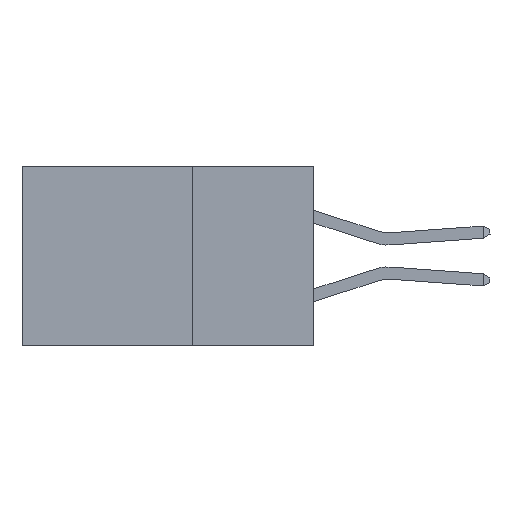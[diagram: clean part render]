
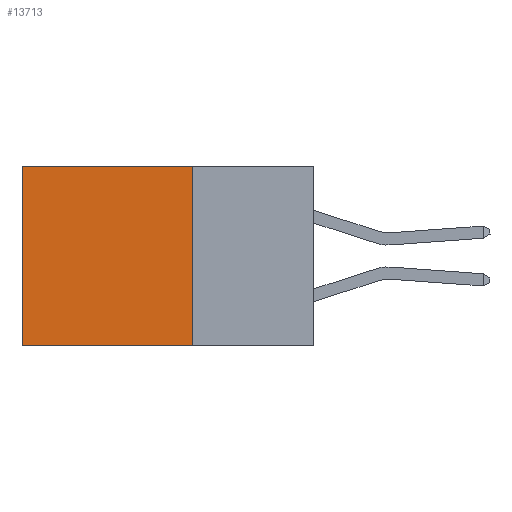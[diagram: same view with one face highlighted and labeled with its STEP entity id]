
A CAD part, left-side view. The second image highlights one B-rep face of the part: STEP entity #13713.
In plain terms, the highlighted planar face has unit normal (-1, 0, 0).
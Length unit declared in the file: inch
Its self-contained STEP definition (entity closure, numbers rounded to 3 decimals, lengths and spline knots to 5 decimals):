
#926 = AXIS2_PLACEMENT_3D ( 'NONE', #6875, #1882, #4405 ) ;
#1078 = CARTESIAN_POINT ( 'NONE',  ( 0.2875, 0.25, 0. ) ) ;
#1113 = LINE ( 'NONE', #6274, #14352 ) ;
#1529 = CARTESIAN_POINT ( 'NONE',  ( 0.2875, 0.25, 0. ) ) ;
#1715 = EDGE_LOOP ( 'NONE', ( #12429, #14531, #10984, #3574 ) ) ;
#1882 = DIRECTION ( 'NONE',  ( 1., 0., 0. ) ) ;
#1952 = DIRECTION ( 'NONE',  ( 0., 1., 0. ) ) ;
#2621 = EDGE_CURVE ( 'NONE', #4861, #4803, #1113, .T. ) ;
#2750 = LINE ( 'NONE', #1529, #8101 ) ;
#3574 = ORIENTED_EDGE ( 'NONE', *, *, #9240, .T. ) ;
#4405 = DIRECTION ( 'NONE',  ( 0., 0., -1. ) ) ;
#4420 = CARTESIAN_POINT ( 'NONE',  ( 0.2875, 0.25, -0.37 ) ) ;
#4532 = VERTEX_POINT ( 'NONE', #4826 ) ;
#4803 = VERTEX_POINT ( 'NONE', #4420 ) ;
#4826 = CARTESIAN_POINT ( 'NONE',  ( 0.2875, 0.6, 0. ) ) ;
#4861 = VERTEX_POINT ( 'NONE', #1078 ) ;
#6040 = DIRECTION ( 'NONE',  ( 0., 0., -1. ) ) ;
#6274 = CARTESIAN_POINT ( 'NONE',  ( 0.2875, 0.25, 0. ) ) ;
#6792 = FACE_OUTER_BOUND ( 'NONE', #1715, .T. ) ;
#6875 = CARTESIAN_POINT ( 'NONE',  ( 0.2875, 0.25, 0. ) ) ;
#8101 = VECTOR ( 'NONE', #8971, 39.37008 ) ;
#8647 = DIRECTION ( 'NONE',  ( 0., 0., -1. ) ) ;
#8971 = DIRECTION ( 'NONE',  ( 0., 1., 0. ) ) ;
#9240 = EDGE_CURVE ( 'NONE', #4861, #4532, #2750, .T. ) ;
#9966 = VERTEX_POINT ( 'NONE', #12414 ) ;
#10215 = EDGE_CURVE ( 'NONE', #4803, #9966, #15778, .T. ) ;
#10984 = ORIENTED_EDGE ( 'NONE', *, *, #2621, .F. ) ;
#11860 = CARTESIAN_POINT ( 'NONE',  ( 0.2875, 0.25, -0.37 ) ) ;
#11866 = PLANE ( 'NONE',  #926 ) ;
#12026 = VECTOR ( 'NONE', #1952, 39.37008 ) ;
#12414 = CARTESIAN_POINT ( 'NONE',  ( 0.2875, 0.6, -0.37 ) ) ;
#12429 = ORIENTED_EDGE ( 'NONE', *, *, #13860, .T. ) ;
#13445 = LINE ( 'NONE', #14742, #15564 ) ;
#13713 = ADVANCED_FACE ( 'NONE', ( #6792 ), #11866, .F. ) ;
#13860 = EDGE_CURVE ( 'NONE', #4532, #9966, #13445, .T. ) ;
#14352 = VECTOR ( 'NONE', #6040, 39.37008 ) ;
#14531 = ORIENTED_EDGE ( 'NONE', *, *, #10215, .F. ) ;
#14742 = CARTESIAN_POINT ( 'NONE',  ( 0.2875, 0.6, 0. ) ) ;
#15564 = VECTOR ( 'NONE', #8647, 39.37008 ) ;
#15778 = LINE ( 'NONE', #11860, #12026 ) ;
